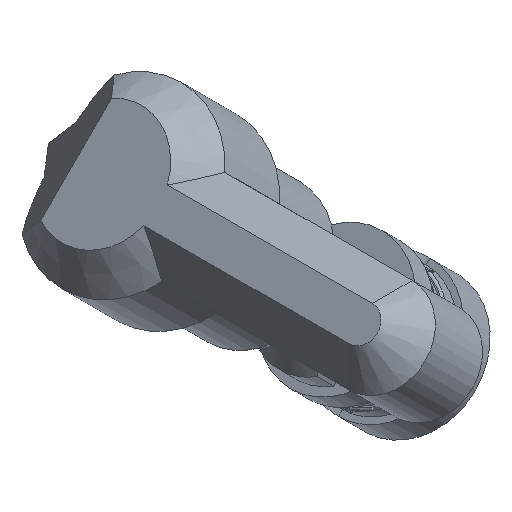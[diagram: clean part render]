
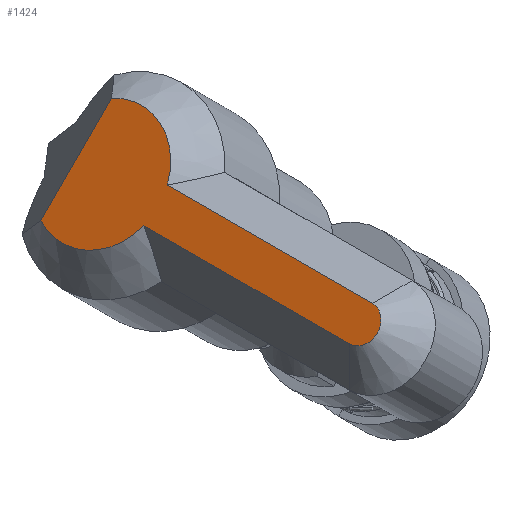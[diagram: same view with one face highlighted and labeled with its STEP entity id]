
A CAD part, isometric view. The second image highlights one B-rep face of the part: STEP entity #1424.
In plain terms, the highlighted planar face has unit normal (-0.707, 0, 0.707).
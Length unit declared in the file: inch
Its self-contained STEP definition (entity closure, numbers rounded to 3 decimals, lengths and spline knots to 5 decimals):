
#60=LINE('',#3190,#135);
#62=LINE('',#3200,#137);
#66=LINE('',#3213,#141);
#135=VECTOR('',#1754,0.3937);
#137=VECTOR('',#1762,0.3937);
#141=VECTOR('',#1774,0.3937);
#229=PLANE('',#1575);
#343=FACE_OUTER_BOUND('',#426,.T.);
#426=EDGE_LOOP('',(#1257,#1258,#1259,#1260,#1261,#1262));
#485=CIRCLE('',#1528,0.15748);
#486=CIRCLE('',#1531,0.04626);
#487=CIRCLE('',#1534,0.15748);
#651=VERTEX_POINT('',#3176);
#652=VERTEX_POINT('',#3180);
#653=VERTEX_POINT('',#3187);
#654=VERTEX_POINT('',#3189);
#655=VERTEX_POINT('',#3196);
#656=VERTEX_POINT('',#3203);
#826=EDGE_CURVE('',#651,#652,#485,.T.);
#829=EDGE_CURVE('',#653,#654,#60,.T.);
#832=EDGE_CURVE('',#655,#653,#486,.T.);
#833=EDGE_CURVE('',#652,#655,#62,.T.);
#835=EDGE_CURVE('',#654,#656,#487,.T.);
#839=EDGE_CURVE('',#651,#656,#66,.T.);
#1257=ORIENTED_EDGE('',*,*,#826,.F.);
#1258=ORIENTED_EDGE('',*,*,#839,.T.);
#1259=ORIENTED_EDGE('',*,*,#835,.F.);
#1260=ORIENTED_EDGE('',*,*,#829,.F.);
#1261=ORIENTED_EDGE('',*,*,#832,.F.);
#1262=ORIENTED_EDGE('',*,*,#833,.F.);
#1424=ADVANCED_FACE('',(#343),#229,.T.);
#1528=AXIS2_PLACEMENT_3D('',#3181,#1749,#1750);
#1531=AXIS2_PLACEMENT_3D('',#3198,#1758,#1759);
#1534=AXIS2_PLACEMENT_3D('',#3204,#1766,#1767);
#1575=AXIS2_PLACEMENT_3D('',#3409,#1877,#1878);
#1749=DIRECTION('center_axis',(0.707,0.,-0.707));
#1750=DIRECTION('ref_axis',(0.707,0.,0.707));
#1754=DIRECTION('',(0.,1.,0.));
#1758=DIRECTION('center_axis',(0.707,0.,-0.707));
#1759=DIRECTION('ref_axis',(-0.707,0.,-0.707));
#1762=DIRECTION('',(0.,-1.,0.));
#1766=DIRECTION('center_axis',(0.707,0.,-0.707));
#1767=DIRECTION('ref_axis',(0.,-1.,0.));
#1774=DIRECTION('',(-0.707,0.,-0.707));
#1877=DIRECTION('center_axis',(-0.707,0.,0.707));
#1878=DIRECTION('ref_axis',(0.,-1.,0.));
#3176=CARTESIAN_POINT('',(-0.09846,0.07219,0.43025));
#3180=CARTESIAN_POINT('',(-0.16471,-0.15053,0.36399));
#3181=CARTESIAN_POINT('Origin',(-0.19742,0.,0.33128));
#3187=CARTESIAN_POINT('',(-0.23013,-0.725,0.29857));
#3189=CARTESIAN_POINT('',(-0.23013,-0.15053,0.29857));
#3190=CARTESIAN_POINT('',(-0.23013,-0.275,0.29857));
#3196=CARTESIAN_POINT('',(-0.16471,-0.725,0.36399));
#3198=CARTESIAN_POINT('Origin',(-0.19742,-0.725,0.33128));
#3200=CARTESIAN_POINT('',(-0.16471,-0.575,0.36399));
#3203=CARTESIAN_POINT('',(-0.29639,0.07219,0.23232));
#3204=CARTESIAN_POINT('Origin',(-0.19742,0.,0.33128));
#3213=CARTESIAN_POINT('',(-0.15323,0.07219,0.37548));
#3409=CARTESIAN_POINT('Origin',(-0.19742,-0.425,0.33128));
